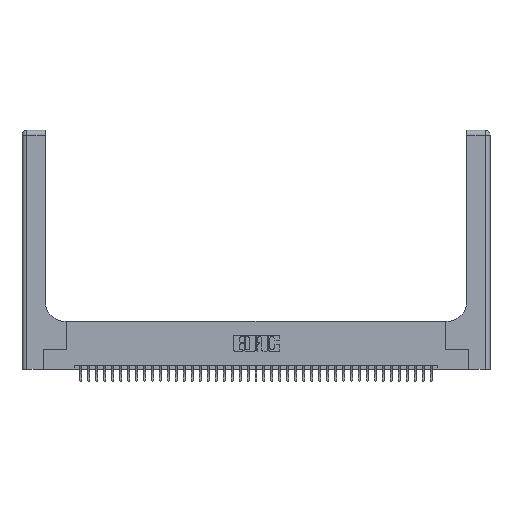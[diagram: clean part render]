
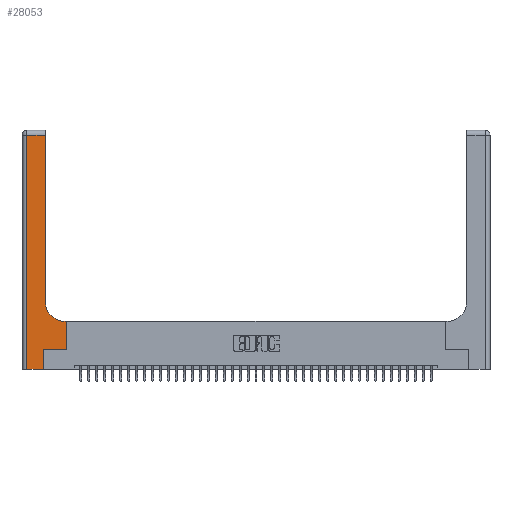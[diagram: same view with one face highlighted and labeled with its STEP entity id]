
A CAD part, top view. The second image highlights one B-rep face of the part: STEP entity #28053.
In plain terms, the highlighted planar face has unit normal (0, 0, 1).
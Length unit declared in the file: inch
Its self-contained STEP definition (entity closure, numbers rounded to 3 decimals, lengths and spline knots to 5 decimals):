
#244 = DIRECTION ( 'NONE',  ( 0., -1., 0. ) ) ;
#1611 = CARTESIAN_POINT ( 'NONE',  ( 0.2915, 0.85, 0.37 ) ) ;
#2375 = EDGE_CURVE ( 'NONE', #13576, #36702, #18892, .T. ) ;
#2505 = CARTESIAN_POINT ( 'NONE',  ( 0.06, 3., 0.37 ) ) ;
#2898 = FACE_OUTER_BOUND ( 'NONE', #30329, .T. ) ;
#3716 = CARTESIAN_POINT ( 'NONE',  ( 0.5585, 0.25, 0.37 ) ) ;
#4057 = LINE ( 'NONE', #30174, #38120 ) ;
#4395 = LINE ( 'NONE', #15549, #36529 ) ;
#4675 = EDGE_CURVE ( 'NONE', #24744, #15643, #10850, .T. ) ;
#5421 = CARTESIAN_POINT ( 'NONE',  ( 0.5415, 0.85, 0.37 ) ) ;
#5911 = VERTEX_POINT ( 'NONE', #1611 ) ;
#6325 = ORIENTED_EDGE ( 'NONE', *, *, #18015, .T. ) ;
#7479 = LINE ( 'NONE', #12476, #16307 ) ;
#8085 = DIRECTION ( 'NONE',  ( 0., 1., 0. ) ) ;
#8834 = DIRECTION ( 'NONE',  ( 1., 0., 0. ) ) ;
#10051 = DIRECTION ( 'NONE',  ( -1., 0., 0. ) ) ;
#10850 = LINE ( 'NONE', #2505, #32272 ) ;
#11208 = ORIENTED_EDGE ( 'NONE', *, *, #2375, .T. ) ;
#11514 = DIRECTION ( 'NONE',  ( -1., 0., 0. ) ) ;
#11882 = VERTEX_POINT ( 'NONE', #39607 ) ;
#12358 = ORIENTED_EDGE ( 'NONE', *, *, #27875, .T. ) ;
#12476 = CARTESIAN_POINT ( 'NONE',  ( 0.269, 0.25, 0.37 ) ) ;
#13576 = VERTEX_POINT ( 'NONE', #18633 ) ;
#14324 = ORIENTED_EDGE ( 'NONE', *, *, #21606, .T. ) ;
#14723 = CIRCLE ( 'NONE', #35935, 0.25 ) ;
#15549 = CARTESIAN_POINT ( 'NONE',  ( 0., 2.94, 0.37 ) ) ;
#15643 = VERTEX_POINT ( 'NONE', #32858 ) ;
#16307 = VECTOR ( 'NONE', #37141, 39.37008 ) ;
#16367 = EDGE_CURVE ( 'NONE', #5911, #27862, #38621, .T. ) ;
#16578 = ORIENTED_EDGE ( 'NONE', *, *, #16367, .T. ) ;
#17016 = ORIENTED_EDGE ( 'NONE', *, *, #4675, .T. ) ;
#18015 = EDGE_CURVE ( 'NONE', #27862, #24744, #4395, .T. ) ;
#18059 = VECTOR ( 'NONE', #31725, 39.37008 ) ;
#18633 = CARTESIAN_POINT ( 'NONE',  ( 0.269, 0., 0.37 ) ) ;
#18892 = LINE ( 'NONE', #26900, #24252 ) ;
#18939 = ORIENTED_EDGE ( 'NONE', *, *, #31767, .T. ) ;
#20970 = AXIS2_PLACEMENT_3D ( 'NONE', #37641, #28644, #23453 ) ;
#21606 = EDGE_CURVE ( 'NONE', #36702, #11882, #7479, .T. ) ;
#21624 = PLANE ( 'NONE',  #20970 ) ;
#21684 = VECTOR ( 'NONE', #21762, 39.37008 ) ;
#21762 = DIRECTION ( 'NONE',  ( 1., 0., 0. ) ) ;
#23453 = DIRECTION ( 'NONE',  ( -1., 0., 0. ) ) ;
#24232 = EDGE_CURVE ( 'NONE', #15643, #13576, #37695, .T. ) ;
#24252 = VECTOR ( 'NONE', #8085, 39.37008 ) ;
#24380 = DIRECTION ( 'NONE',  ( 0., 0., -1. ) ) ;
#24744 = VERTEX_POINT ( 'NONE', #36380 ) ;
#24764 = CARTESIAN_POINT ( 'NONE',  ( 0., 0., 0.37 ) ) ;
#26224 = DIRECTION ( 'NONE',  ( 0., 1., 0. ) ) ;
#26302 = LINE ( 'NONE', #3716, #18059 ) ;
#26900 = CARTESIAN_POINT ( 'NONE',  ( 0.269, 0., 0.37 ) ) ;
#27388 = CARTESIAN_POINT ( 'NONE',  ( 0.5415, 0.6, 0.37 ) ) ;
#27862 = VERTEX_POINT ( 'NONE', #32000 ) ;
#27875 = EDGE_CURVE ( 'NONE', #11882, #38449, #26302, .T. ) ;
#27886 = CARTESIAN_POINT ( 'NONE',  ( 0.269, 0.25, 0.37 ) ) ;
#28053 = ADVANCED_FACE ( 'NONE', ( #2898 ), #21624, .F. ) ;
#28100 = ORIENTED_EDGE ( 'NONE', *, *, #24232, .T. ) ;
#28644 = DIRECTION ( 'NONE',  ( 0., 0., -1. ) ) ;
#29451 = CARTESIAN_POINT ( 'NONE',  ( 0.5585, 0.6, 0.37 ) ) ;
#30174 = CARTESIAN_POINT ( 'NONE',  ( 0.2915, 0.6, 0.37 ) ) ;
#30329 = EDGE_LOOP ( 'NONE', ( #16578, #6325, #17016, #28100, #11208, #14324, #12358, #38924, #18939 ) ) ;
#31725 = DIRECTION ( 'NONE',  ( 0., 1., 0. ) ) ;
#31767 = EDGE_CURVE ( 'NONE', #34641, #5911, #14723, .T. ) ;
#32000 = CARTESIAN_POINT ( 'NONE',  ( 0.2915, 2.94, 0.37 ) ) ;
#32272 = VECTOR ( 'NONE', #244, 39.37008 ) ;
#32858 = CARTESIAN_POINT ( 'NONE',  ( 0.06, 0., 0.37 ) ) ;
#33004 = CARTESIAN_POINT ( 'NONE',  ( 0.2915, 3., 0.37 ) ) ;
#33757 = VECTOR ( 'NONE', #26224, 39.37008 ) ;
#34641 = VERTEX_POINT ( 'NONE', #27388 ) ;
#35935 = AXIS2_PLACEMENT_3D ( 'NONE', #5421, #24380, #8834 ) ;
#36380 = CARTESIAN_POINT ( 'NONE',  ( 0.06, 2.94, 0.37 ) ) ;
#36529 = VECTOR ( 'NONE', #10051, 39.37008 ) ;
#36702 = VERTEX_POINT ( 'NONE', #27886 ) ;
#37141 = DIRECTION ( 'NONE',  ( 1., 0., 0. ) ) ;
#37641 = CARTESIAN_POINT ( 'NONE',  ( 0., 3., 0.37 ) ) ;
#37695 = LINE ( 'NONE', #24764, #21684 ) ;
#38120 = VECTOR ( 'NONE', #11514, 39.37008 ) ;
#38449 = VERTEX_POINT ( 'NONE', #29451 ) ;
#38621 = LINE ( 'NONE', #33004, #33757 ) ;
#38924 = ORIENTED_EDGE ( 'NONE', *, *, #39974, .T. ) ;
#39607 = CARTESIAN_POINT ( 'NONE',  ( 0.5585, 0.25, 0.37 ) ) ;
#39974 = EDGE_CURVE ( 'NONE', #38449, #34641, #4057, .T. ) ;
